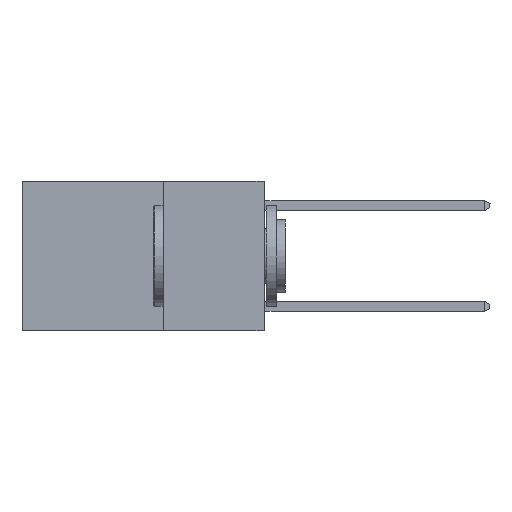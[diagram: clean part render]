
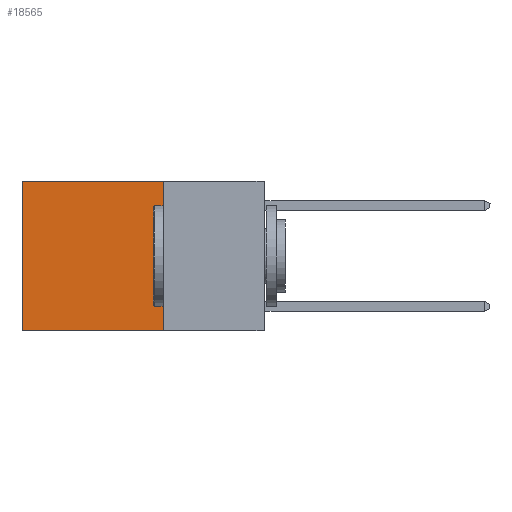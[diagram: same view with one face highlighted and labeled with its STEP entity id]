
A CAD part, left-side view. The second image highlights one B-rep face of the part: STEP entity #18565.
In plain terms, the highlighted planar face has unit normal (-1, 0, 0).
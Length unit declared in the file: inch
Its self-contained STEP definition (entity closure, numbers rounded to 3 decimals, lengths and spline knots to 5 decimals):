
#621 = VECTOR ( 'NONE', #30338, 39.37008 ) ;
#1331 = EDGE_CURVE ( 'NONE', #17059, #5463, #30570, .T. ) ;
#1877 = CARTESIAN_POINT ( 'NONE',  ( 0.2625, 0.25, -0.37 ) ) ;
#3746 = DIRECTION ( 'NONE',  ( 0., 0., -1. ) ) ;
#3759 = LINE ( 'NONE', #15290, #621 ) ;
#3870 = VECTOR ( 'NONE', #3746, 39.37008 ) ;
#5258 = CARTESIAN_POINT ( 'NONE',  ( 0.2625, 0.25, 0. ) ) ;
#5463 = VERTEX_POINT ( 'NONE', #19453 ) ;
#5671 = ORIENTED_EDGE ( 'NONE', *, *, #24249, .T. ) ;
#9195 = FACE_OUTER_BOUND ( 'NONE', #22196, .T. ) ;
#9475 = LINE ( 'NONE', #1877, #11780 ) ;
#11645 = CARTESIAN_POINT ( 'NONE',  ( 0.2625, 0.25, 0. ) ) ;
#11780 = VECTOR ( 'NONE', #14378, 39.37008 ) ;
#12437 = VERTEX_POINT ( 'NONE', #20244 ) ;
#13558 = DIRECTION ( 'NONE',  ( 1., 0., 0. ) ) ;
#14236 = CARTESIAN_POINT ( 'NONE',  ( 0.2625, 0.25, 0. ) ) ;
#14378 = DIRECTION ( 'NONE',  ( 0., 1., 0. ) ) ;
#15246 = LINE ( 'NONE', #23786, #3870 ) ;
#15290 = CARTESIAN_POINT ( 'NONE',  ( 0.2625, 0.25, 0. ) ) ;
#15569 = CARTESIAN_POINT ( 'NONE',  ( 0.2625, 0.6, 0. ) ) ;
#15669 = ORIENTED_EDGE ( 'NONE', *, *, #1331, .F. ) ;
#16487 = EDGE_CURVE ( 'NONE', #17059, #17725, #3759, .T. ) ;
#17059 = VERTEX_POINT ( 'NONE', #14236 ) ;
#17389 = VECTOR ( 'NONE', #22679, 39.37008 ) ;
#17449 = AXIS2_PLACEMENT_3D ( 'NONE', #11645, #13558, #21965 ) ;
#17725 = VERTEX_POINT ( 'NONE', #15569 ) ;
#18565 = ADVANCED_FACE ( 'NONE', ( #9195 ), #21101, .F. ) ;
#19453 = CARTESIAN_POINT ( 'NONE',  ( 0.2625, 0.25, -0.37 ) ) ;
#20244 = CARTESIAN_POINT ( 'NONE',  ( 0.2625, 0.6, -0.37 ) ) ;
#21101 = PLANE ( 'NONE',  #17449 ) ;
#21965 = DIRECTION ( 'NONE',  ( 0., 0., -1. ) ) ;
#22072 = ORIENTED_EDGE ( 'NONE', *, *, #16487, .T. ) ;
#22196 = EDGE_LOOP ( 'NONE', ( #5671, #31763, #15669, #22072 ) ) ;
#22679 = DIRECTION ( 'NONE',  ( 0., 0., -1. ) ) ;
#23078 = EDGE_CURVE ( 'NONE', #5463, #12437, #9475, .T. ) ;
#23786 = CARTESIAN_POINT ( 'NONE',  ( 0.2625, 0.6, 0. ) ) ;
#24249 = EDGE_CURVE ( 'NONE', #17725, #12437, #15246, .T. ) ;
#30338 = DIRECTION ( 'NONE',  ( 0., 1., 0. ) ) ;
#30570 = LINE ( 'NONE', #5258, #17389 ) ;
#31763 = ORIENTED_EDGE ( 'NONE', *, *, #23078, .F. ) ;
